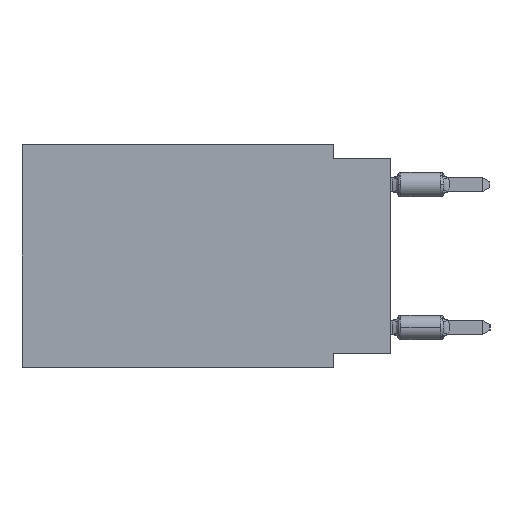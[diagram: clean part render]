
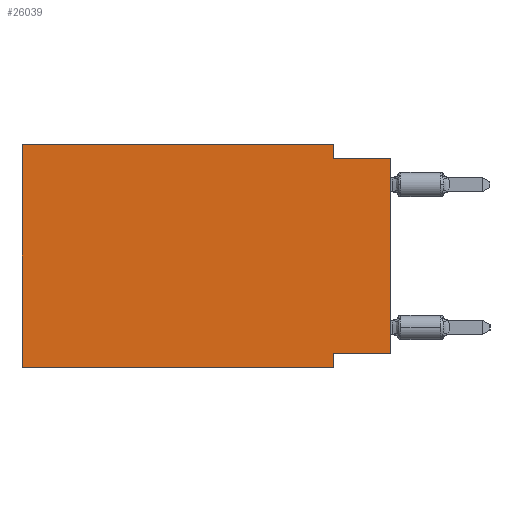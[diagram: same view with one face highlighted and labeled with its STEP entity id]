
A CAD part, left-side view. The second image highlights one B-rep face of the part: STEP entity #26039.
In plain terms, the highlighted planar face has unit normal (-1, 0, 0).
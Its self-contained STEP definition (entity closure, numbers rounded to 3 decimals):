
#392 = VECTOR ( 'NONE', #17830, 1000. ) ;
#747 = VECTOR ( 'NONE', #20225, 1000. ) ;
#1409 = DIRECTION ( 'NONE',  ( 1., 0., 0. ) ) ;
#1607 = EDGE_CURVE ( 'NONE', #22715, #17361, #16377, .T. ) ;
#1742 = CARTESIAN_POINT ( 'NONE',  ( 0., 2.54, 0. ) ) ;
#2130 = VECTOR ( 'NONE', #9632, 1000. ) ;
#2266 = DIRECTION ( 'NONE',  ( 0., 0., 1. ) ) ;
#3832 = VECTOR ( 'NONE', #22382, 1000. ) ;
#4253 = ORIENTED_EDGE ( 'NONE', *, *, #23890, .F. ) ;
#4505 = CARTESIAN_POINT ( 'NONE',  ( 0., 2.54, -9.906 ) ) ;
#5028 = CARTESIAN_POINT ( 'NONE',  ( 0., 16.383, -9.906 ) ) ;
#5096 = EDGE_CURVE ( 'NONE', #6330, #22715, #13680, .T. ) ;
#5502 = FACE_OUTER_BOUND ( 'NONE', #6990, .T. ) ;
#5967 = CARTESIAN_POINT ( 'NONE',  ( 0., 16.383, 0. ) ) ;
#6069 = CARTESIAN_POINT ( 'NONE',  ( 0., 16.383, 0. ) ) ;
#6330 = VERTEX_POINT ( 'NONE', #12673 ) ;
#6607 = VERTEX_POINT ( 'NONE', #18522 ) ;
#6888 = VECTOR ( 'NONE', #15503, 1000. ) ;
#6990 = EDGE_LOOP ( 'NONE', ( #20563, #19028, #15856, #4253, #26458, #8423, #23903, #8528 ) ) ;
#7854 = LINE ( 'NONE', #5967, #392 ) ;
#8053 = VERTEX_POINT ( 'NONE', #5028 ) ;
#8082 = CARTESIAN_POINT ( 'NONE',  ( 0., 16.383, -9.906 ) ) ;
#8423 = ORIENTED_EDGE ( 'NONE', *, *, #8828, .T. ) ;
#8528 = ORIENTED_EDGE ( 'NONE', *, *, #5096, .F. ) ;
#8828 = EDGE_CURVE ( 'NONE', #8053, #17361, #24599, .T. ) ;
#9141 = CARTESIAN_POINT ( 'NONE',  ( 0., 2.54, -0.635 ) ) ;
#9572 = DIRECTION ( 'NONE',  ( 0., 0., -1. ) ) ;
#9632 = DIRECTION ( 'NONE',  ( 0., 0., -1. ) ) ;
#9826 = LINE ( 'NONE', #16104, #3832 ) ;
#10133 = EDGE_CURVE ( 'NONE', #8053, #19133, #20095, .T. ) ;
#12031 = CARTESIAN_POINT ( 'NONE',  ( 0., 16.383, 0. ) ) ;
#12287 = CARTESIAN_POINT ( 'NONE',  ( 0., 2.54, -9.906 ) ) ;
#12590 = CARTESIAN_POINT ( 'NONE',  ( 0., 0., 0. ) ) ;
#12673 = CARTESIAN_POINT ( 'NONE',  ( 0., 0., -9.271 ) ) ;
#12810 = VECTOR ( 'NONE', #22806, 1000. ) ;
#13680 = LINE ( 'NONE', #22038, #6888 ) ;
#14347 = VERTEX_POINT ( 'NONE', #18293 ) ;
#15503 = DIRECTION ( 'NONE',  ( 0., 1., 0. ) ) ;
#15856 = ORIENTED_EDGE ( 'NONE', *, *, #23947, .F. ) ;
#16104 = CARTESIAN_POINT ( 'NONE',  ( 0., 0., -0.635 ) ) ;
#16377 = LINE ( 'NONE', #12287, #12810 ) ;
#17071 = VECTOR ( 'NONE', #18599, 1000. ) ;
#17361 = VERTEX_POINT ( 'NONE', #4505 ) ;
#17830 = DIRECTION ( 'NONE',  ( 0., -1., 0. ) ) ;
#18034 = EDGE_CURVE ( 'NONE', #6330, #14347, #20924, .T. ) ;
#18293 = CARTESIAN_POINT ( 'NONE',  ( 0., 0., -0.635 ) ) ;
#18522 = CARTESIAN_POINT ( 'NONE',  ( 0., 2.54, 0. ) ) ;
#18599 = DIRECTION ( 'NONE',  ( 0., -1., 0. ) ) ;
#19028 = ORIENTED_EDGE ( 'NONE', *, *, #23131, .F. ) ;
#19133 = VERTEX_POINT ( 'NONE', #6069 ) ;
#20095 = LINE ( 'NONE', #12031, #747 ) ;
#20225 = DIRECTION ( 'NONE',  ( 0., 0., 1. ) ) ;
#20563 = ORIENTED_EDGE ( 'NONE', *, *, #18034, .T. ) ;
#20789 = CARTESIAN_POINT ( 'NONE',  ( 0., 2.54, -9.271 ) ) ;
#20924 = LINE ( 'NONE', #12590, #24218 ) ;
#22038 = CARTESIAN_POINT ( 'NONE',  ( 0., 0., -9.271 ) ) ;
#22187 = LINE ( 'NONE', #1742, #2130 ) ;
#22382 = DIRECTION ( 'NONE',  ( 0., -1., 0. ) ) ;
#22715 = VERTEX_POINT ( 'NONE', #20789 ) ;
#22806 = DIRECTION ( 'NONE',  ( 0., 0., -1. ) ) ;
#23131 = EDGE_CURVE ( 'NONE', #23442, #14347, #9826, .T. ) ;
#23442 = VERTEX_POINT ( 'NONE', #9141 ) ;
#23890 = EDGE_CURVE ( 'NONE', #19133, #6607, #7854, .T. ) ;
#23903 = ORIENTED_EDGE ( 'NONE', *, *, #1607, .F. ) ;
#23947 = EDGE_CURVE ( 'NONE', #6607, #23442, #22187, .T. ) ;
#24218 = VECTOR ( 'NONE', #2266, 1000. ) ;
#24599 = LINE ( 'NONE', #8082, #17071 ) ;
#25948 = AXIS2_PLACEMENT_3D ( 'NONE', #26253, #1409, #9572 ) ;
#26039 = ADVANCED_FACE ( 'NONE', ( #5502 ), #26380, .F. ) ;
#26253 = CARTESIAN_POINT ( 'NONE',  ( 0., 16.383, 0. ) ) ;
#26380 = PLANE ( 'NONE',  #25948 ) ;
#26458 = ORIENTED_EDGE ( 'NONE', *, *, #10133, .F. ) ;
